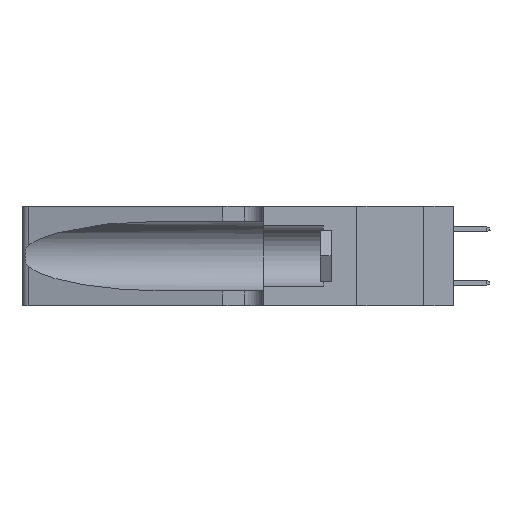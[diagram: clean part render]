
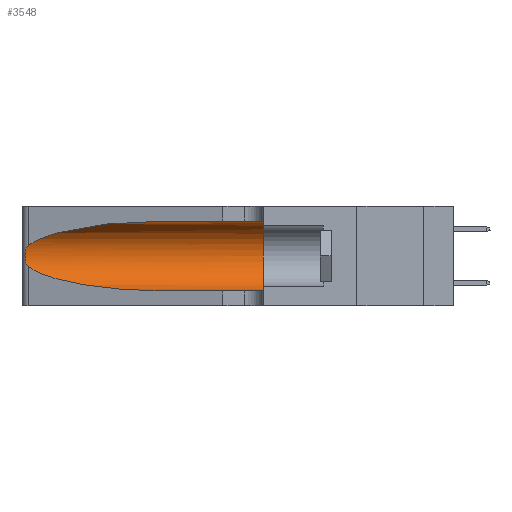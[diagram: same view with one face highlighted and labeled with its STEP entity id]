
A CAD part, left-side view. The second image highlights one B-rep face of the part: STEP entity #3548.
In plain terms, the highlighted cylindrical face has radius 3.308 mm (diameter 6.617 mm), a partial arc.
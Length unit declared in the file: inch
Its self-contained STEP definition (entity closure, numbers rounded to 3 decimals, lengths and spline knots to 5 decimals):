
#1143 = AXIS2_PLACEMENT_3D ( 'NONE', #10034, #9805, #44716 ) ;
#3022 =( BOUNDED_CURVE ( )  B_SPLINE_CURVE ( 3, ( #21186, #25065, #28720, #41952 ),
 .UNSPECIFIED., .F., .F. ) 
 B_SPLINE_CURVE_WITH_KNOTS ( ( 4, 4 ),
 ( 1.5708, 2.84003 ),
 .UNSPECIFIED. ) 
 CURVE ( )  GEOMETRIC_REPRESENTATION_ITEM ( )  RATIONAL_B_SPLINE_CURVE ( ( 1., 0.87, 0.87, 1. ) ) 
 REPRESENTATION_ITEM ( '' )  );
#3058 = VERTEX_POINT ( 'NONE', #12428 ) ;
#3534 = CARTESIAN_POINT ( 'NONE',  ( 0.26018, 1.23835, 0.19895 ) ) ;
#3548 = ADVANCED_FACE ( 'NONE', ( #44511 ), #41316, .F. ) ;
#5492 = CARTESIAN_POINT ( 'NONE',  ( 0.1305, 0.35, 0.05475 ) ) ;
#6506 = CARTESIAN_POINT ( 'NONE',  ( 0.25856, 1.23593, 0.16098 ) ) ;
#7074 = AXIS2_PLACEMENT_3D ( 'NONE', #42172, #41279, #44905 ) ;
#7261 = LINE ( 'NONE', #25349, #19377 ) ;
#8515 = CARTESIAN_POINT ( 'NONE',  ( 0.1305, 0.72297, 0.05475 ) ) ;
#9732 = CARTESIAN_POINT ( 'NONE',  ( 0.25487, 1.22718, 0.22369 ) ) ;
#9805 = DIRECTION ( 'NONE',  ( 0., -1., 0. ) ) ;
#9966 = CARTESIAN_POINT ( 'NONE',  ( 0.25555, 1.22994, 0.2215 ) ) ;
#10034 = CARTESIAN_POINT ( 'NONE',  ( 0.1305, 1.61858, 0.185 ) ) ;
#10498 = CARTESIAN_POINT ( 'NONE',  ( 0.25487, 1.22718, 0.22369 ) ) ;
#10645 = CARTESIAN_POINT ( 'NONE',  ( 0.25639, 1.23184, 0.21858 ) ) ;
#11058 = EDGE_CURVE ( 'NONE', #29796, #19144, #11514, .T. ) ;
#11136 = ORIENTED_EDGE ( 'NONE', *, *, #20129, .T. ) ;
#11514 = CIRCLE ( 'NONE', #7074, 0.13025 ) ;
#11763 = CARTESIAN_POINT ( 'NONE',  ( 0.2373, 1.15595, 0.08982 ) ) ;
#12428 = CARTESIAN_POINT ( 'NONE',  ( 0.1305, 0.72297, 0.05475 ) ) ;
#17033 = CARTESIAN_POINT ( 'NONE',  ( 0.25854, 1.2359, 0.20912 ) ) ;
#17456 = CARTESIAN_POINT ( 'NONE',  ( 0.1305, 0.35, 0.31525 ) ) ;
#19094 = B_SPLINE_CURVE_WITH_KNOTS ( 'NONE', 3,
 ( #9732, #9966, #10645, #24583, #17033, #3534, #38500, #23911, #37818, #6506, #20464, #30958, #44873, #31414 ),
 .UNSPECIFIED., .F., .F.,
 ( 4, 2, 2, 2, 2, 2, 4 ),
 ( 0., 0.00027, 0.00053, 0.00107, 0.0016, 0.00187, 0.00214 ),
 .UNSPECIFIED. ) ;
#19144 = VERTEX_POINT ( 'NONE', #5492 ) ;
#19332 = LINE ( 'NONE', #43747, #44386 ) ;
#19377 = VECTOR ( 'NONE', #39269, 39.37008 ) ;
#20129 = EDGE_CURVE ( 'NONE', #25299, #33562, #3022, .T. ) ;
#20464 = CARTESIAN_POINT ( 'NONE',  ( 0.25789, 1.23486, 0.15765 ) ) ;
#21186 = CARTESIAN_POINT ( 'NONE',  ( 0.1305, 0.72297, 0.31525 ) ) ;
#23276 = EDGE_CURVE ( 'NONE', #33562, #28954, #19094, .T. ) ;
#23911 = CARTESIAN_POINT ( 'NONE',  ( 0.26075, 1.23896, 0.178 ) ) ;
#23989 = CARTESIAN_POINT ( 'NONE',  ( 0.25487, 1.22718, 0.14631 ) ) ;
#24501 = EDGE_LOOP ( 'NONE', ( #11136, #41302, #28376, #44388, #28057, #36938 ) ) ;
#24583 = CARTESIAN_POINT ( 'NONE',  ( 0.25787, 1.23484, 0.2124 ) ) ;
#25065 = CARTESIAN_POINT ( 'NONE',  ( 0.18966, 0.96281, 0.31525 ) ) ;
#25299 = VERTEX_POINT ( 'NONE', #32284 ) ;
#25349 = CARTESIAN_POINT ( 'NONE',  ( 0.1305, 1.61858, 0.05475 ) ) ;
#25456 = CARTESIAN_POINT ( 'NONE',  ( 0.18966, 0.96281, 0.05475 ) ) ;
#28057 = ORIENTED_EDGE ( 'NONE', *, *, #11058, .F. ) ;
#28376 = ORIENTED_EDGE ( 'NONE', *, *, #31354, .T. ) ;
#28414 = CARTESIAN_POINT ( 'NONE',  ( 0.25487, 1.22718, 0.14631 ) ) ;
#28720 = CARTESIAN_POINT ( 'NONE',  ( 0.2373, 1.15595, 0.28018 ) ) ;
#28954 = VERTEX_POINT ( 'NONE', #23989 ) ;
#29796 = VERTEX_POINT ( 'NONE', #17456 ) ;
#30958 = CARTESIAN_POINT ( 'NONE',  ( 0.25639, 1.23186, 0.15144 ) ) ;
#31354 = EDGE_CURVE ( 'NONE', #28954, #3058, #38666, .T. ) ;
#31414 = CARTESIAN_POINT ( 'NONE',  ( 0.25487, 1.22718, 0.14631 ) ) ;
#32284 = CARTESIAN_POINT ( 'NONE',  ( 0.1305, 0.72297, 0.31525 ) ) ;
#32847 = EDGE_CURVE ( 'NONE', #25299, #29796, #19332, .T. ) ;
#33562 = VERTEX_POINT ( 'NONE', #10498 ) ;
#36913 = DIRECTION ( 'NONE',  ( 0., -1., 0. ) ) ;
#36938 = ORIENTED_EDGE ( 'NONE', *, *, #32847, .F. ) ;
#37818 = CARTESIAN_POINT ( 'NONE',  ( 0.26017, 1.23833, 0.17102 ) ) ;
#38500 = CARTESIAN_POINT ( 'NONE',  ( 0.26075, 1.23896, 0.19203 ) ) ;
#38666 =( BOUNDED_CURVE ( )  B_SPLINE_CURVE ( 3, ( #28414, #11763, #25456, #8515 ),
 .UNSPECIFIED., .F., .F. ) 
 B_SPLINE_CURVE_WITH_KNOTS ( ( 4, 4 ),
 ( 3.44316, 4.71239 ),
 .UNSPECIFIED. ) 
 CURVE ( )  GEOMETRIC_REPRESENTATION_ITEM ( )  RATIONAL_B_SPLINE_CURVE ( ( 1., 0.87, 0.87, 1. ) ) 
 REPRESENTATION_ITEM ( '' )  );
#39269 = DIRECTION ( 'NONE',  ( 0., -1., 0. ) ) ;
#39340 = EDGE_CURVE ( 'NONE', #3058, #19144, #7261, .T. ) ;
#41279 = DIRECTION ( 'NONE',  ( 0., 1., 0. ) ) ;
#41302 = ORIENTED_EDGE ( 'NONE', *, *, #23276, .T. ) ;
#41316 = CYLINDRICAL_SURFACE ( 'NONE', #1143, 0.13025 ) ;
#41952 = CARTESIAN_POINT ( 'NONE',  ( 0.25487, 1.22718, 0.22369 ) ) ;
#42172 = CARTESIAN_POINT ( 'NONE',  ( 0.1305, 0.35, 0.185 ) ) ;
#43747 = CARTESIAN_POINT ( 'NONE',  ( 0.1305, 1.61858, 0.31525 ) ) ;
#44386 = VECTOR ( 'NONE', #36913, 39.37008 ) ;
#44388 = ORIENTED_EDGE ( 'NONE', *, *, #39340, .T. ) ;
#44511 = FACE_OUTER_BOUND ( 'NONE', #24501, .T. ) ;
#44716 = DIRECTION ( 'NONE',  ( 0., 0., -1. ) ) ;
#44873 = CARTESIAN_POINT ( 'NONE',  ( 0.25555, 1.22993, 0.14849 ) ) ;
#44905 = DIRECTION ( 'NONE',  ( 0., 0., 1. ) ) ;
